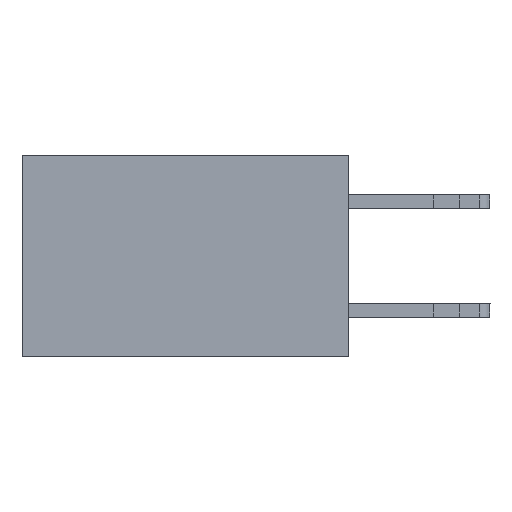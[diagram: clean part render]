
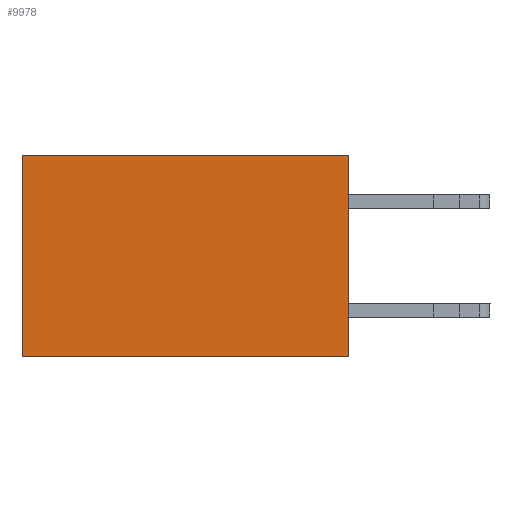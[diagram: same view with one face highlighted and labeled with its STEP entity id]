
A CAD part, left-side view. The second image highlights one B-rep face of the part: STEP entity #9978.
In plain terms, the highlighted planar face has unit normal (-1, 0, 0).
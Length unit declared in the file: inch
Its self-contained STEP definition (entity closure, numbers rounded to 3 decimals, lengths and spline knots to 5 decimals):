
#313 = LINE ( 'NONE', #12562, #7400 ) ;
#355 = VECTOR ( 'NONE', #10689, 39.37008 ) ;
#942 = EDGE_CURVE ( 'NONE', #8843, #11254, #14809, .T. ) ;
#1952 = LINE ( 'NONE', #2768, #16237 ) ;
#2751 = CARTESIAN_POINT ( 'NONE',  ( 0.2615, 0., -0.37 ) ) ;
#2768 = CARTESIAN_POINT ( 'NONE',  ( 0.2615, 0.6, -0.37 ) ) ;
#2859 = CARTESIAN_POINT ( 'NONE',  ( 0.2615, 0., -0.37 ) ) ;
#3973 = ORIENTED_EDGE ( 'NONE', *, *, #942, .F. ) ;
#4903 = LINE ( 'NONE', #12806, #11566 ) ;
#5462 = FACE_OUTER_BOUND ( 'NONE', #9572, .T. ) ;
#5727 = ORIENTED_EDGE ( 'NONE', *, *, #7612, .T. ) ;
#5957 = DIRECTION ( 'NONE',  ( 0., 1., 0. ) ) ;
#7036 = CARTESIAN_POINT ( 'NONE',  ( 0.2615, 0., -0.37 ) ) ;
#7400 = VECTOR ( 'NONE', #5957, 39.37008 ) ;
#7612 = EDGE_CURVE ( 'NONE', #8843, #16728, #313, .T. ) ;
#8843 = VERTEX_POINT ( 'NONE', #9928 ) ;
#9297 = CARTESIAN_POINT ( 'NONE',  ( 0.2615, 0.6, -0.37 ) ) ;
#9572 = EDGE_LOOP ( 'NONE', ( #14553, #13642, #3973, #5727 ) ) ;
#9642 = DIRECTION ( 'NONE',  ( 0., 0., -1. ) ) ;
#9928 = CARTESIAN_POINT ( 'NONE',  ( 0.2615, 0., 0. ) ) ;
#9978 = ADVANCED_FACE ( 'NONE', ( #5462 ), #10916, .F. ) ;
#10689 = DIRECTION ( 'NONE',  ( 0., 0., -1. ) ) ;
#10847 = CARTESIAN_POINT ( 'NONE',  ( 0.2615, 0.6, 0. ) ) ;
#10916 = PLANE ( 'NONE',  #15491 ) ;
#11254 = VERTEX_POINT ( 'NONE', #2859 ) ;
#11566 = VECTOR ( 'NONE', #14143, 39.37008 ) ;
#12235 = DIRECTION ( 'NONE',  ( 0., 0., -1. ) ) ;
#12562 = CARTESIAN_POINT ( 'NONE',  ( 0.2615, 0., 0. ) ) ;
#12806 = CARTESIAN_POINT ( 'NONE',  ( 0.2615, 0., -0.37 ) ) ;
#13642 = ORIENTED_EDGE ( 'NONE', *, *, #15868, .F. ) ;
#14143 = DIRECTION ( 'NONE',  ( 0., 1., 0. ) ) ;
#14448 = VERTEX_POINT ( 'NONE', #9297 ) ;
#14553 = ORIENTED_EDGE ( 'NONE', *, *, #16223, .T. ) ;
#14809 = LINE ( 'NONE', #2751, #355 ) ;
#15491 = AXIS2_PLACEMENT_3D ( 'NONE', #7036, #17431, #9642 ) ;
#15868 = EDGE_CURVE ( 'NONE', #11254, #14448, #4903, .T. ) ;
#16223 = EDGE_CURVE ( 'NONE', #16728, #14448, #1952, .T. ) ;
#16237 = VECTOR ( 'NONE', #12235, 39.37008 ) ;
#16728 = VERTEX_POINT ( 'NONE', #10847 ) ;
#17431 = DIRECTION ( 'NONE',  ( 1., 0., 0. ) ) ;
